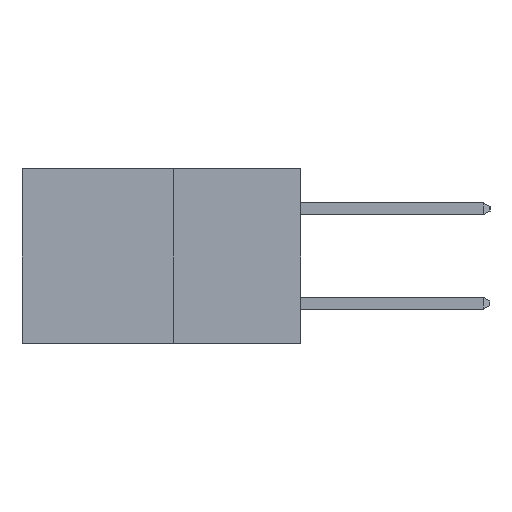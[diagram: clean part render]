
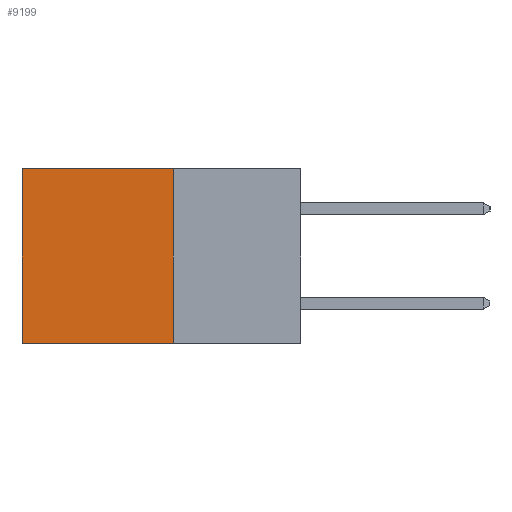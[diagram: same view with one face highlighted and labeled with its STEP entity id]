
A CAD part, left-side view. The second image highlights one B-rep face of the part: STEP entity #9199.
In plain terms, the highlighted planar face has unit normal (-1, 0, 0).
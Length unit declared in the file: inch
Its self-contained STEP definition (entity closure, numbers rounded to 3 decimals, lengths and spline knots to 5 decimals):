
#1854 = DIRECTION ( 'NONE',  ( 0., 1., 0. ) ) ;
#2101 = LINE ( 'NONE', #13105, #19419 ) ;
#3241 = LINE ( 'NONE', #3777, #3952 ) ;
#3756 = EDGE_CURVE ( 'NONE', #24606, #11055, #3241, .T. ) ;
#3777 = CARTESIAN_POINT ( 'NONE',  ( 0.277, 0.59, -0.37 ) ) ;
#3952 = VECTOR ( 'NONE', #25134, 39.37008 ) ;
#5147 = DIRECTION ( 'NONE',  ( 0., 1., 0. ) ) ;
#5526 = DIRECTION ( 'NONE',  ( 1., 0., 0. ) ) ;
#6875 = PLANE ( 'NONE',  #17548 ) ;
#6991 = CARTESIAN_POINT ( 'NONE',  ( 0.277, 0.59, -0.37 ) ) ;
#7661 = VERTEX_POINT ( 'NONE', #18155 ) ;
#7870 = VECTOR ( 'NONE', #22518, 39.37008 ) ;
#8683 = DIRECTION ( 'NONE',  ( 0., 0., -1. ) ) ;
#9025 = CARTESIAN_POINT ( 'NONE',  ( 0.277, 0.27, -0.37 ) ) ;
#9199 = ADVANCED_FACE ( 'NONE', ( #23276 ), #6875, .F. ) ;
#9447 = ORIENTED_EDGE ( 'NONE', *, *, #3756, .T. ) ;
#9808 = CARTESIAN_POINT ( 'NONE',  ( 0.277, 0.27, -0.37 ) ) ;
#10573 = EDGE_CURVE ( 'NONE', #22070, #11055, #22489, .T. ) ;
#11055 = VERTEX_POINT ( 'NONE', #6991 ) ;
#11158 = CARTESIAN_POINT ( 'NONE',  ( 0.277, 0.59, 0. ) ) ;
#11283 = ORIENTED_EDGE ( 'NONE', *, *, #13181, .F. ) ;
#11437 = EDGE_LOOP ( 'NONE', ( #9447, #25108, #11283, #22699 ) ) ;
#13105 = CARTESIAN_POINT ( 'NONE',  ( 0.277, 0.27, 0. ) ) ;
#13181 = EDGE_CURVE ( 'NONE', #7661, #22070, #13876, .T. ) ;
#13876 = LINE ( 'NONE', #9025, #7870 ) ;
#16515 = VECTOR ( 'NONE', #5147, 39.37008 ) ;
#17548 = AXIS2_PLACEMENT_3D ( 'NONE', #24226, #5526, #8683 ) ;
#18155 = CARTESIAN_POINT ( 'NONE',  ( 0.277, 0.27, 0. ) ) ;
#19419 = VECTOR ( 'NONE', #1854, 39.37008 ) ;
#22070 = VERTEX_POINT ( 'NONE', #9808 ) ;
#22489 = LINE ( 'NONE', #25280, #16515 ) ;
#22518 = DIRECTION ( 'NONE',  ( 0., 0., -1. ) ) ;
#22699 = ORIENTED_EDGE ( 'NONE', *, *, #27392, .T. ) ;
#23276 = FACE_OUTER_BOUND ( 'NONE', #11437, .T. ) ;
#24226 = CARTESIAN_POINT ( 'NONE',  ( 0.277, 0.27, -0.37 ) ) ;
#24606 = VERTEX_POINT ( 'NONE', #11158 ) ;
#25108 = ORIENTED_EDGE ( 'NONE', *, *, #10573, .F. ) ;
#25134 = DIRECTION ( 'NONE',  ( 0., 0., -1. ) ) ;
#25280 = CARTESIAN_POINT ( 'NONE',  ( 0.277, 0.27, -0.37 ) ) ;
#27392 = EDGE_CURVE ( 'NONE', #7661, #24606, #2101, .T. ) ;
